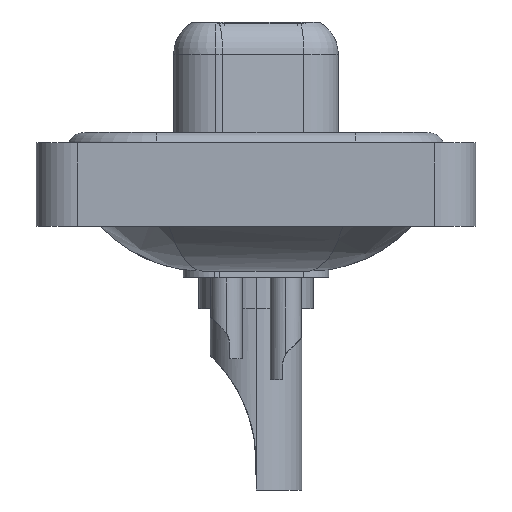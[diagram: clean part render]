
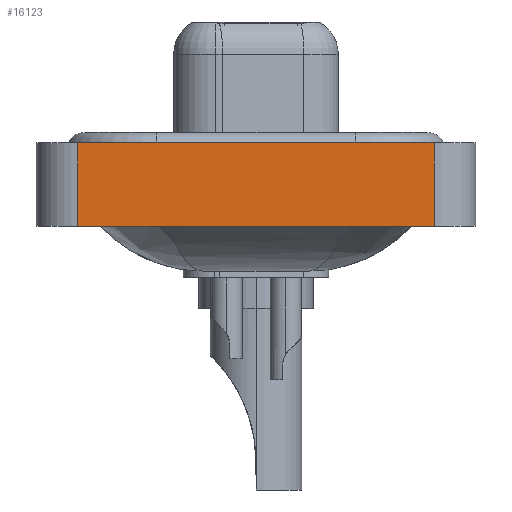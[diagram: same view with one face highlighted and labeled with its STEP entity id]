
A CAD part, left-side view. The second image highlights one B-rep face of the part: STEP entity #16123.
In plain terms, the highlighted planar face has unit normal (-1, 0, 0).
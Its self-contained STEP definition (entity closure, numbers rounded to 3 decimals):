
#771 = LINE ( 'NONE', #11940, #9118 ) ;
#1977 = EDGE_CURVE ( 'NONE', #4011, #19009, #6385, .T. ) ;
#2125 = ORIENTED_EDGE ( 'NONE', *, *, #1977, .T. ) ;
#3272 = VECTOR ( 'NONE', #12364, 1000. ) ;
#3477 = CARTESIAN_POINT ( 'NONE',  ( -7.25, -8.55, 0.4 ) ) ;
#4011 = VERTEX_POINT ( 'NONE', #7242 ) ;
#4179 = VECTOR ( 'NONE', #6589, 1000. ) ;
#4618 = DIRECTION ( 'NONE',  ( -1., 0., 0. ) ) ;
#5145 = EDGE_CURVE ( 'NONE', #19009, #7190, #771, .T. ) ;
#5426 = EDGE_LOOP ( 'NONE', ( #14387, #8161, #7292, #2125 ) ) ;
#6259 = FACE_OUTER_BOUND ( 'NONE', #5426, .T. ) ;
#6385 = LINE ( 'NONE', #8130, #4179 ) ;
#6589 = DIRECTION ( 'NONE',  ( 0., -1., 0. ) ) ;
#6630 = CARTESIAN_POINT ( 'NONE',  ( -7.25, -8.55, -3.6 ) ) ;
#7190 = VERTEX_POINT ( 'NONE', #3477 ) ;
#7242 = CARTESIAN_POINT ( 'NONE',  ( -7.25, 8.55, -3.6 ) ) ;
#7292 = ORIENTED_EDGE ( 'NONE', *, *, #13617, .F. ) ;
#8130 = CARTESIAN_POINT ( 'NONE',  ( -7.25, -8.55, -3.6 ) ) ;
#8161 = ORIENTED_EDGE ( 'NONE', *, *, #8928, .F. ) ;
#8928 = EDGE_CURVE ( 'NONE', #10652, #7190, #12565, .T. ) ;
#9118 = VECTOR ( 'NONE', #14801, 1000. ) ;
#9210 = DIRECTION ( 'NONE',  ( 0., 0., 1. ) ) ;
#10652 = VERTEX_POINT ( 'NONE', #16875 ) ;
#10862 = DIRECTION ( 'NONE',  ( 0., 0., 1. ) ) ;
#11166 = PLANE ( 'NONE',  #14859 ) ;
#11940 = CARTESIAN_POINT ( 'NONE',  ( -7.25, -8.55, -3.6 ) ) ;
#12083 = LINE ( 'NONE', #18438, #18009 ) ;
#12364 = DIRECTION ( 'NONE',  ( 0., -1., 0. ) ) ;
#12565 = LINE ( 'NONE', #20152, #3272 ) ;
#12905 = CARTESIAN_POINT ( 'NONE',  ( -7.25, -8.55, -3.6 ) ) ;
#13617 = EDGE_CURVE ( 'NONE', #4011, #10652, #12083, .T. ) ;
#14387 = ORIENTED_EDGE ( 'NONE', *, *, #5145, .T. ) ;
#14801 = DIRECTION ( 'NONE',  ( 0., 0., 1. ) ) ;
#14859 = AXIS2_PLACEMENT_3D ( 'NONE', #12905, #4618, #10862 ) ;
#16123 = ADVANCED_FACE ( 'NONE', ( #6259 ), #11166, .T. ) ;
#16875 = CARTESIAN_POINT ( 'NONE',  ( -7.25, 8.55, 0.4 ) ) ;
#18009 = VECTOR ( 'NONE', #9210, 1000. ) ;
#18438 = CARTESIAN_POINT ( 'NONE',  ( -7.25, 8.55, -3.6 ) ) ;
#19009 = VERTEX_POINT ( 'NONE', #6630 ) ;
#20152 = CARTESIAN_POINT ( 'NONE',  ( -7.25, -8.55, 0.4 ) ) ;
